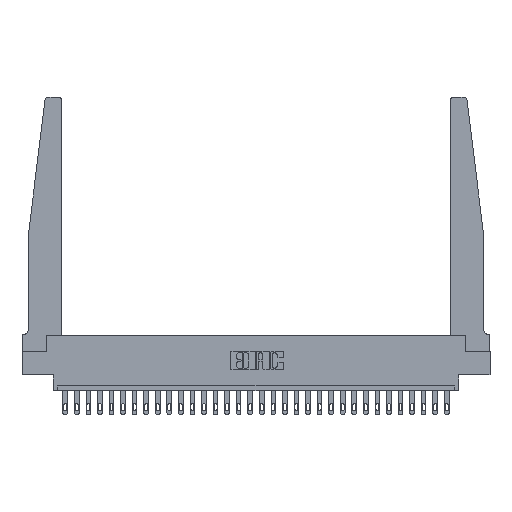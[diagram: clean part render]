
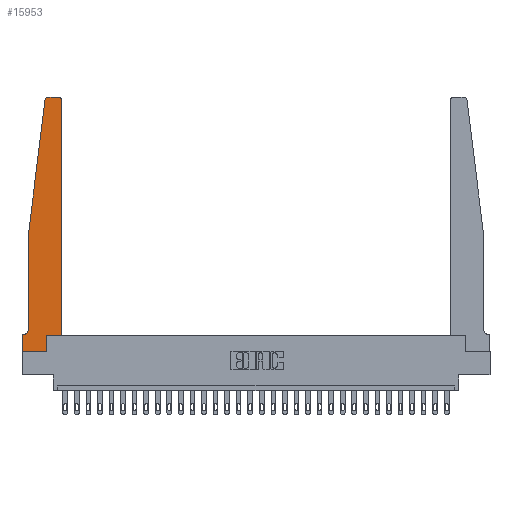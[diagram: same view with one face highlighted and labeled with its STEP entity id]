
A CAD part, top view. The second image highlights one B-rep face of the part: STEP entity #15953.
In plain terms, the highlighted planar face has unit normal (0, 0, 1).
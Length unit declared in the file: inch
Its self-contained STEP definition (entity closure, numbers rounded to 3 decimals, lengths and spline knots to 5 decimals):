
#503 = CARTESIAN_POINT ( 'NONE',  ( 0., 0.1875, 0.37 ) ) ;
#768 = DIRECTION ( 'NONE',  ( 1., 0., 0. ) ) ;
#863 = EDGE_CURVE ( 'NONE', #985, #2069, #25964, .T. ) ;
#985 = VERTEX_POINT ( 'NONE', #26383 ) ;
#1576 = ORIENTED_EDGE ( 'NONE', *, *, #6912, .T. ) ;
#1592 = EDGE_CURVE ( 'NONE', #13094, #3003, #26654, .T. ) ;
#1637 = CARTESIAN_POINT ( 'NONE',  ( 0.065, 1.25, 0.37 ) ) ;
#2000 = EDGE_CURVE ( 'NONE', #3003, #4599, #18232, .T. ) ;
#2069 = VERTEX_POINT ( 'NONE', #26860 ) ;
#2248 = VECTOR ( 'NONE', #2773, 39.37008 ) ;
#2320 = ORIENTED_EDGE ( 'NONE', *, *, #6727, .T. ) ;
#2411 = CARTESIAN_POINT ( 'NONE',  ( 0.015, 0.2375, 0.37 ) ) ;
#2773 = DIRECTION ( 'NONE',  ( -0.122, -0.992, 0. ) ) ;
#3003 = VERTEX_POINT ( 'NONE', #12628 ) ;
#3115 = DIRECTION ( 'NONE',  ( 0., 0., 1. ) ) ;
#3620 = VERTEX_POINT ( 'NONE', #19353 ) ;
#3641 = ORIENTED_EDGE ( 'NONE', *, *, #20579, .T. ) ;
#3908 = DIRECTION ( 'NONE',  ( 0., 0., 1. ) ) ;
#3989 = AXIS2_PLACEMENT_3D ( 'NONE', #23076, #3908, #16942 ) ;
#4161 = CARTESIAN_POINT ( 'NONE',  ( 0.25, 2.75, 0.37 ) ) ;
#4217 = ORIENTED_EDGE ( 'NONE', *, *, #19822, .T. ) ;
#4449 = VERTEX_POINT ( 'NONE', #16183 ) ;
#4599 = VERTEX_POINT ( 'NONE', #23391 ) ;
#4738 = EDGE_CURVE ( 'NONE', #3620, #22963, #19496, .T. ) ;
#5194 = DIRECTION ( 'NONE',  ( 0., 1., 0. ) ) ;
#5364 = VERTEX_POINT ( 'NONE', #20851 ) ;
#6207 = DIRECTION ( 'NONE',  ( 0., 0., -1. ) ) ;
#6523 = DIRECTION ( 'NONE',  ( -1., 0., 0. ) ) ;
#6622 = CARTESIAN_POINT ( 'NONE',  ( 0., 0., 0.37 ) ) ;
#6648 = CARTESIAN_POINT ( 'NONE',  ( 0., 0., 0.37 ) ) ;
#6727 = EDGE_CURVE ( 'NONE', #15627, #13094, #23182, .T. ) ;
#6831 = VERTEX_POINT ( 'NONE', #6648 ) ;
#6912 = EDGE_CURVE ( 'NONE', #2069, #6831, #27307, .T. ) ;
#7022 = AXIS2_PLACEMENT_3D ( 'NONE', #2411, #6207, #23134 ) ;
#7036 = VECTOR ( 'NONE', #5194, 39.37008 ) ;
#8373 = ORIENTED_EDGE ( 'NONE', *, *, #1592, .T. ) ;
#8412 = ORIENTED_EDGE ( 'NONE', *, *, #4738, .T. ) ;
#8812 = CARTESIAN_POINT ( 'NONE',  ( 0.2605, 0.18, 0.37 ) ) ;
#9086 = PLANE ( 'NONE',  #17162 ) ;
#9300 = VECTOR ( 'NONE', #19543, 39.37008 ) ;
#9879 = LINE ( 'NONE', #22665, #26162 ) ;
#10077 = DIRECTION ( 'NONE',  ( 0., -1., 0. ) ) ;
#10114 = CARTESIAN_POINT ( 'NONE',  ( 0.395, 2.75, 0.37 ) ) ;
#10231 = CARTESIAN_POINT ( 'NONE',  ( 0.27653, 2.72, 0.37 ) ) ;
#10643 = VERTEX_POINT ( 'NONE', #24121 ) ;
#10768 = DIRECTION ( 'NONE',  ( 1., 0., 0. ) ) ;
#11017 = VECTOR ( 'NONE', #10768, 39.37008 ) ;
#12181 = DIRECTION ( 'NONE',  ( 0., 0., 1. ) ) ;
#12209 = LINE ( 'NONE', #1637, #14497 ) ;
#12628 = CARTESIAN_POINT ( 'NONE',  ( 0.24675, 2.72367, 0.37 ) ) ;
#12756 = EDGE_CURVE ( 'NONE', #22963, #4449, #26026, .T. ) ;
#13094 = VERTEX_POINT ( 'NONE', #21254 ) ;
#13222 = CIRCLE ( 'NONE', #7022, 0.05 ) ;
#14497 = VECTOR ( 'NONE', #22755, 39.37008 ) ;
#14661 = AXIS2_PLACEMENT_3D ( 'NONE', #10231, #12181, #27180 ) ;
#15418 = ORIENTED_EDGE ( 'NONE', *, *, #12756, .T. ) ;
#15533 = CARTESIAN_POINT ( 'NONE',  ( 0.065, 1.25, 0.37 ) ) ;
#15559 = VECTOR ( 'NONE', #10077, 39.37008 ) ;
#15627 = VERTEX_POINT ( 'NONE', #10114 ) ;
#15638 = EDGE_CURVE ( 'NONE', #4599, #5364, #12209, .T. ) ;
#15681 = ORIENTED_EDGE ( 'NONE', *, *, #15638, .T. ) ;
#15691 = ORIENTED_EDGE ( 'NONE', *, *, #17261, .T. ) ;
#15953 = ADVANCED_FACE ( 'NONE', ( #17973 ), #9086, .T. ) ;
#16183 = CARTESIAN_POINT ( 'NONE',  ( 0.425, 0.18, 0.37 ) ) ;
#16344 = ORIENTED_EDGE ( 'NONE', *, *, #20370, .T. ) ;
#16942 = DIRECTION ( 'NONE',  ( 1., 0., 0. ) ) ;
#17162 = AXIS2_PLACEMENT_3D ( 'NONE', #503, #3115, #768 ) ;
#17261 = EDGE_CURVE ( 'NONE', #5364, #985, #13222, .T. ) ;
#17674 = DIRECTION ( 'NONE',  ( 1., 0., 0. ) ) ;
#17890 = ORIENTED_EDGE ( 'NONE', *, *, #863, .T. ) ;
#17973 = FACE_OUTER_BOUND ( 'NONE', #23317, .T. ) ;
#18072 = CARTESIAN_POINT ( 'NONE',  ( 0.425, 0.18, 0.37 ) ) ;
#18232 = LINE ( 'NONE', #15533, #2248 ) ;
#18339 = DIRECTION ( 'NONE',  ( 0., 1., 0. ) ) ;
#18808 = CARTESIAN_POINT ( 'NONE',  ( 0., 0., 0.37 ) ) ;
#19353 = CARTESIAN_POINT ( 'NONE',  ( 0.2605, 0., 0.37 ) ) ;
#19496 = LINE ( 'NONE', #8812, #7036 ) ;
#19543 = DIRECTION ( 'NONE',  ( -1., 0., 0. ) ) ;
#19822 = EDGE_CURVE ( 'NONE', #6831, #3620, #23972, .T. ) ;
#19930 = CIRCLE ( 'NONE', #3989, 0.03 ) ;
#20071 = VECTOR ( 'NONE', #6523, 39.37008 ) ;
#20222 = ORIENTED_EDGE ( 'NONE', *, *, #2000, .T. ) ;
#20370 = EDGE_CURVE ( 'NONE', #4449, #10643, #9879, .T. ) ;
#20579 = EDGE_CURVE ( 'NONE', #10643, #15627, #19930, .T. ) ;
#20851 = CARTESIAN_POINT ( 'NONE',  ( 0.065, 0.2375, 0.37 ) ) ;
#21254 = CARTESIAN_POINT ( 'NONE',  ( 0.27653, 2.75, 0.37 ) ) ;
#21447 = VECTOR ( 'NONE', #17674, 39.37008 ) ;
#22665 = CARTESIAN_POINT ( 'NONE',  ( 0.425, 0.18, 0.37 ) ) ;
#22755 = DIRECTION ( 'NONE',  ( 0., -1., 0. ) ) ;
#22963 = VERTEX_POINT ( 'NONE', #25706 ) ;
#23076 = CARTESIAN_POINT ( 'NONE',  ( 0.395, 2.72, 0.37 ) ) ;
#23134 = DIRECTION ( 'NONE',  ( -1., 0., 0. ) ) ;
#23182 = LINE ( 'NONE', #4161, #9300 ) ;
#23317 = EDGE_LOOP ( 'NONE', ( #2320, #8373, #20222, #15681, #15691, #17890, #1576, #4217, #8412, #15418, #16344, #3641 ) ) ;
#23391 = CARTESIAN_POINT ( 'NONE',  ( 0.065, 1.25, 0.37 ) ) ;
#23972 = LINE ( 'NONE', #6622, #11017 ) ;
#24121 = CARTESIAN_POINT ( 'NONE',  ( 0.425, 2.72, 0.37 ) ) ;
#25545 = CARTESIAN_POINT ( 'NONE',  ( 0.065, 0.1875, 0.37 ) ) ;
#25706 = CARTESIAN_POINT ( 'NONE',  ( 0.2605, 0.18, 0.37 ) ) ;
#25964 = LINE ( 'NONE', #25545, #20071 ) ;
#26026 = LINE ( 'NONE', #18072, #21447 ) ;
#26162 = VECTOR ( 'NONE', #18339, 39.37008 ) ;
#26383 = CARTESIAN_POINT ( 'NONE',  ( 0.015, 0.1875, 0.37 ) ) ;
#26654 = CIRCLE ( 'NONE', #14661, 0.03 ) ;
#26860 = CARTESIAN_POINT ( 'NONE',  ( 0., 0.1875, 0.37 ) ) ;
#27180 = DIRECTION ( 'NONE',  ( 1., 0., 0. ) ) ;
#27307 = LINE ( 'NONE', #18808, #15559 ) ;
